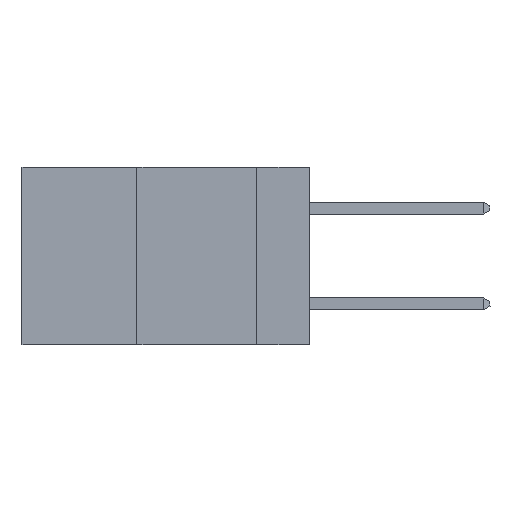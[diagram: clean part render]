
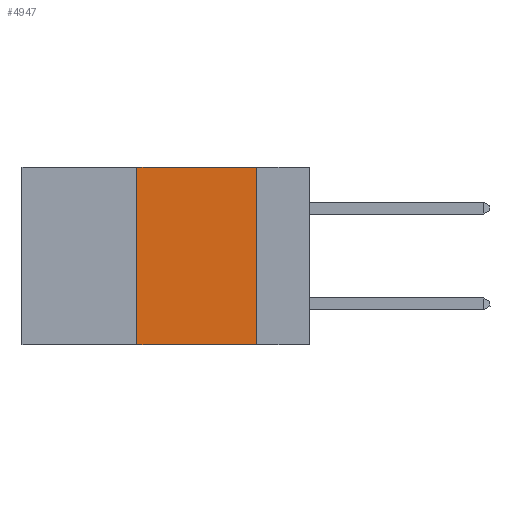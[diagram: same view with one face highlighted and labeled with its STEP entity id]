
A CAD part, left-side view. The second image highlights one B-rep face of the part: STEP entity #4947.
In plain terms, the highlighted planar face has unit normal (-1, 0, 0).
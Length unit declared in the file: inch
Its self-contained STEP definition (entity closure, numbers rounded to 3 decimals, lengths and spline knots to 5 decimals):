
#2010 = EDGE_CURVE ( 'NONE', #3060, #12165, #22430, .T. ) ;
#2031 = CARTESIAN_POINT ( 'NONE',  ( 0., 0.11, -0.37 ) ) ;
#2388 = CARTESIAN_POINT ( 'NONE',  ( 0., 0.36, -0.37 ) ) ;
#2583 = EDGE_LOOP ( 'NONE', ( #23244, #21087, #4502, #11437 ) ) ;
#2675 = AXIS2_PLACEMENT_3D ( 'NONE', #23243, #25212, #11638 ) ;
#3060 = VERTEX_POINT ( 'NONE', #2388 ) ;
#3357 = FACE_OUTER_BOUND ( 'NONE', #2583, .T. ) ;
#3574 = DIRECTION ( 'NONE',  ( 0., -1., 0. ) ) ;
#4502 = ORIENTED_EDGE ( 'NONE', *, *, #2010, .F. ) ;
#4613 = LINE ( 'NONE', #23429, #10706 ) ;
#4820 = VECTOR ( 'NONE', #11707, 39.37008 ) ;
#4947 = ADVANCED_FACE ( 'NONE', ( #3357 ), #9591, .F. ) ;
#5304 = VERTEX_POINT ( 'NONE', #2031 ) ;
#7366 = CARTESIAN_POINT ( 'NONE',  ( 0., 0.6, -0.37 ) ) ;
#8060 = DIRECTION ( 'NONE',  ( 0., 0., 1. ) ) ;
#9591 = PLANE ( 'NONE',  #2675 ) ;
#10211 = VECTOR ( 'NONE', #8060, 39.37008 ) ;
#10706 = VECTOR ( 'NONE', #21638, 39.37008 ) ;
#11437 = ORIENTED_EDGE ( 'NONE', *, *, #14637, .T. ) ;
#11638 = DIRECTION ( 'NONE',  ( 0., 0., -1. ) ) ;
#11707 = DIRECTION ( 'NONE',  ( 0., -1., 0. ) ) ;
#12165 = VERTEX_POINT ( 'NONE', #13138 ) ;
#13138 = CARTESIAN_POINT ( 'NONE',  ( 0., 0.36, 0. ) ) ;
#13595 = CARTESIAN_POINT ( 'NONE',  ( 0., 0.6, 0. ) ) ;
#13937 = EDGE_CURVE ( 'NONE', #19286, #5304, #4613, .T. ) ;
#14637 = EDGE_CURVE ( 'NONE', #3060, #5304, #21083, .T. ) ;
#17839 = EDGE_CURVE ( 'NONE', #12165, #19286, #18882, .T. ) ;
#18882 = LINE ( 'NONE', #13595, #4820 ) ;
#19286 = VERTEX_POINT ( 'NONE', #24765 ) ;
#19756 = CARTESIAN_POINT ( 'NONE',  ( 0., 0.36, 0. ) ) ;
#20474 = VECTOR ( 'NONE', #3574, 39.37008 ) ;
#21083 = LINE ( 'NONE', #7366, #20474 ) ;
#21087 = ORIENTED_EDGE ( 'NONE', *, *, #17839, .F. ) ;
#21638 = DIRECTION ( 'NONE',  ( 0., 0., -1. ) ) ;
#22430 = LINE ( 'NONE', #19756, #10211 ) ;
#23243 = CARTESIAN_POINT ( 'NONE',  ( 0., 0.6, 0. ) ) ;
#23244 = ORIENTED_EDGE ( 'NONE', *, *, #13937, .F. ) ;
#23429 = CARTESIAN_POINT ( 'NONE',  ( 0., 0.11, 0. ) ) ;
#24765 = CARTESIAN_POINT ( 'NONE',  ( 0., 0.11, 0. ) ) ;
#25212 = DIRECTION ( 'NONE',  ( 1., 0., 0. ) ) ;
